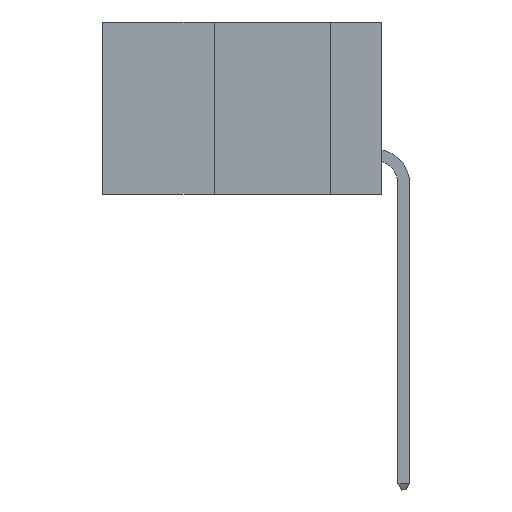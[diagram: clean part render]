
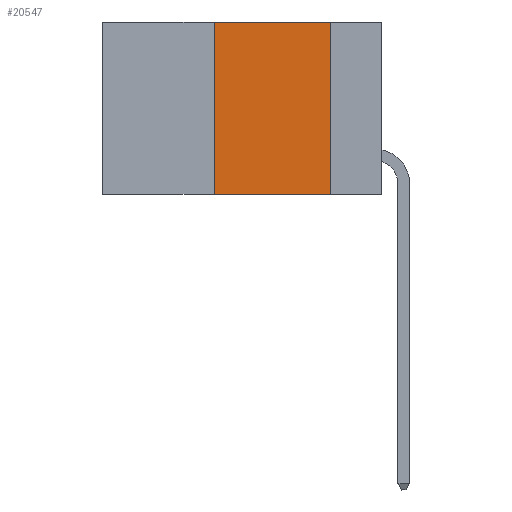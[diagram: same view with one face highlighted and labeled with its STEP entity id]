
A CAD part, left-side view. The second image highlights one B-rep face of the part: STEP entity #20547.
In plain terms, the highlighted planar face has unit normal (-1, 0, 0).
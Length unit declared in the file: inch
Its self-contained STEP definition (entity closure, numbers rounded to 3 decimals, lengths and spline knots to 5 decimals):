
#200 = AXIS2_PLACEMENT_3D ( 'NONE', #11551, #11203, #27992 ) ;
#749 = EDGE_CURVE ( 'NONE', #25872, #34999, #8877, .T. ) ;
#1764 = ORIENTED_EDGE ( 'NONE', *, *, #749, .F. ) ;
#1780 = VERTEX_POINT ( 'NONE', #4091 ) ;
#3542 = EDGE_LOOP ( 'NONE', ( #1764, #23029, #19914, #31538 ) ) ;
#4091 = CARTESIAN_POINT ( 'NONE',  ( 0., 0.36, -0.37 ) ) ;
#6145 = LINE ( 'NONE', #12346, #34964 ) ;
#6482 = CARTESIAN_POINT ( 'NONE',  ( 0., 0.36, 0. ) ) ;
#8068 = CARTESIAN_POINT ( 'NONE',  ( 0., 0.6, 0. ) ) ;
#8624 = CARTESIAN_POINT ( 'NONE',  ( 0., 0.11, -0.37 ) ) ;
#8877 = LINE ( 'NONE', #35799, #22414 ) ;
#9367 = VECTOR ( 'NONE', #29763, 39.37008 ) ;
#11203 = DIRECTION ( 'NONE',  ( 1., 0., 0. ) ) ;
#11551 = CARTESIAN_POINT ( 'NONE',  ( 0., 0.6, 0. ) ) ;
#12346 = CARTESIAN_POINT ( 'NONE',  ( 0., 0.36, 0. ) ) ;
#13202 = VERTEX_POINT ( 'NONE', #6482 ) ;
#14028 = PLANE ( 'NONE',  #200 ) ;
#16326 = CARTESIAN_POINT ( 'NONE',  ( 0., 0.6, -0.37 ) ) ;
#17021 = VECTOR ( 'NONE', #32604, 39.37008 ) ;
#19211 = LINE ( 'NONE', #16326, #17021 ) ;
#19914 = ORIENTED_EDGE ( 'NONE', *, *, #32113, .F. ) ;
#20547 = ADVANCED_FACE ( 'NONE', ( #23251 ), #14028, .F. ) ;
#20759 = DIRECTION ( 'NONE',  ( 0., 0., 1. ) ) ;
#22414 = VECTOR ( 'NONE', #33234, 39.37008 ) ;
#23029 = ORIENTED_EDGE ( 'NONE', *, *, #26294, .F. ) ;
#23251 = FACE_OUTER_BOUND ( 'NONE', #3542, .T. ) ;
#25872 = VERTEX_POINT ( 'NONE', #33867 ) ;
#26294 = EDGE_CURVE ( 'NONE', #13202, #25872, #30744, .T. ) ;
#27992 = DIRECTION ( 'NONE',  ( 0., 0., -1. ) ) ;
#29763 = DIRECTION ( 'NONE',  ( 0., -1., 0. ) ) ;
#30744 = LINE ( 'NONE', #8068, #9367 ) ;
#31538 = ORIENTED_EDGE ( 'NONE', *, *, #35467, .T. ) ;
#32113 = EDGE_CURVE ( 'NONE', #1780, #13202, #6145, .T. ) ;
#32604 = DIRECTION ( 'NONE',  ( 0., -1., 0. ) ) ;
#33234 = DIRECTION ( 'NONE',  ( 0., 0., -1. ) ) ;
#33867 = CARTESIAN_POINT ( 'NONE',  ( 0., 0.11, 0. ) ) ;
#34964 = VECTOR ( 'NONE', #20759, 39.37008 ) ;
#34999 = VERTEX_POINT ( 'NONE', #8624 ) ;
#35467 = EDGE_CURVE ( 'NONE', #1780, #34999, #19211, .T. ) ;
#35799 = CARTESIAN_POINT ( 'NONE',  ( 0., 0.11, 0. ) ) ;
